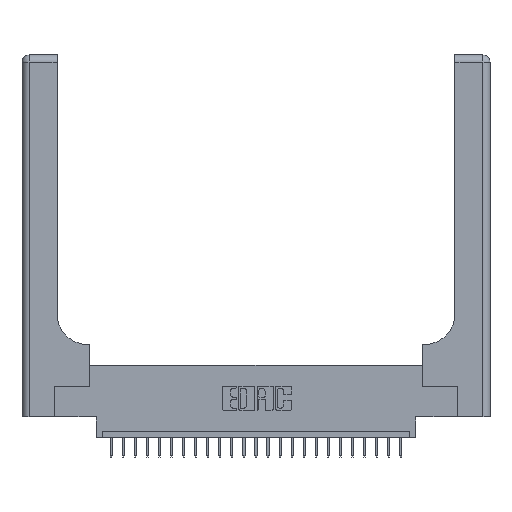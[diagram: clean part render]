
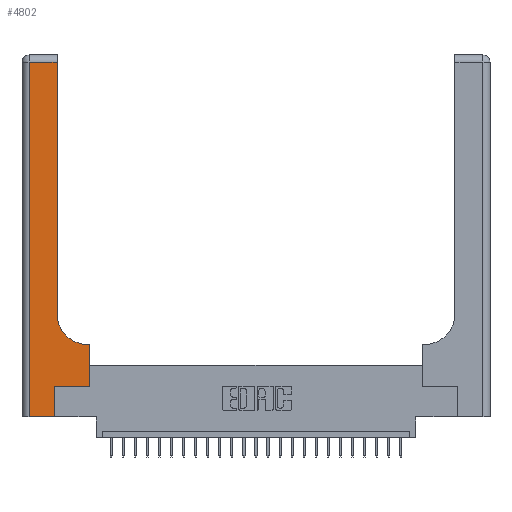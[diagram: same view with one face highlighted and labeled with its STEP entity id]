
A CAD part, top view. The second image highlights one B-rep face of the part: STEP entity #4802.
In plain terms, the highlighted planar face has unit normal (0, 0, 1).
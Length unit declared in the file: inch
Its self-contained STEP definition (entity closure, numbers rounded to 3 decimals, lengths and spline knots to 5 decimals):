
#202 = VERTEX_POINT ( 'NONE', #8876 ) ;
#686 = CARTESIAN_POINT ( 'NONE',  ( 0.06, 2.94, 0.37 ) ) ;
#2284 = DIRECTION ( 'NONE',  ( 0., 1., 0. ) ) ;
#2621 = DIRECTION ( 'NONE',  ( 0., 0., -1. ) ) ;
#2882 = PLANE ( 'NONE',  #21151 ) ;
#2911 = VERTEX_POINT ( 'NONE', #7952 ) ;
#3058 = DIRECTION ( 'NONE',  ( -1., 0., 0. ) ) ;
#3122 = ORIENTED_EDGE ( 'NONE', *, *, #18862, .T. ) ;
#3989 = VERTEX_POINT ( 'NONE', #17909 ) ;
#4230 = VERTEX_POINT ( 'NONE', #686 ) ;
#4232 = CIRCLE ( 'NONE', #15058, 0.25 ) ;
#4802 = ADVANCED_FACE ( 'NONE', ( #13613 ), #2882, .F. ) ;
#5008 = VECTOR ( 'NONE', #9974, 39.37008 ) ;
#5128 = EDGE_CURVE ( 'NONE', #3989, #202, #18696, .T. ) ;
#5741 = VERTEX_POINT ( 'NONE', #21146 ) ;
#6477 = VERTEX_POINT ( 'NONE', #24338 ) ;
#6773 = EDGE_CURVE ( 'NONE', #14384, #8627, #12584, .T. ) ;
#7535 = ORIENTED_EDGE ( 'NONE', *, *, #15723, .T. ) ;
#7834 = LINE ( 'NONE', #13498, #24083 ) ;
#7952 = CARTESIAN_POINT ( 'NONE',  ( 0.5415, 0.6, 0.37 ) ) ;
#8627 = VERTEX_POINT ( 'NONE', #24743 ) ;
#8790 = CARTESIAN_POINT ( 'NONE',  ( 0.5415, 0.85, 0.37 ) ) ;
#8876 = CARTESIAN_POINT ( 'NONE',  ( 0.5585, 0.25, 0.37 ) ) ;
#9069 = VECTOR ( 'NONE', #22063, 39.37008 ) ;
#9974 = DIRECTION ( 'NONE',  ( 0., 1., 0. ) ) ;
#10156 = VERTEX_POINT ( 'NONE', #11970 ) ;
#11117 = VECTOR ( 'NONE', #19999, 39.37008 ) ;
#11348 = VECTOR ( 'NONE', #23626, 39.37008 ) ;
#11970 = CARTESIAN_POINT ( 'NONE',  ( 0.5585, 0.6, 0.37 ) ) ;
#12013 = CARTESIAN_POINT ( 'NONE',  ( 0.06, 3., 0.37 ) ) ;
#12401 = LINE ( 'NONE', #12013, #11117 ) ;
#12412 = ORIENTED_EDGE ( 'NONE', *, *, #6773, .T. ) ;
#12584 = LINE ( 'NONE', #16720, #23110 ) ;
#13239 = CARTESIAN_POINT ( 'NONE',  ( 0., 3., 0.37 ) ) ;
#13437 = ORIENTED_EDGE ( 'NONE', *, *, #14209, .T. ) ;
#13498 = CARTESIAN_POINT ( 'NONE',  ( 0.2915, 0.6, 0.37 ) ) ;
#13613 = FACE_OUTER_BOUND ( 'NONE', #20439, .T. ) ;
#13622 = DIRECTION ( 'NONE',  ( -1., 0., 0. ) ) ;
#13705 = LINE ( 'NONE', #20097, #22325 ) ;
#14209 = EDGE_CURVE ( 'NONE', #4230, #5741, #12401, .T. ) ;
#14384 = VERTEX_POINT ( 'NONE', #24270 ) ;
#14474 = LINE ( 'NONE', #19800, #9069 ) ;
#14749 = EDGE_CURVE ( 'NONE', #6477, #3989, #19337, .T. ) ;
#14861 = ORIENTED_EDGE ( 'NONE', *, *, #26100, .T. ) ;
#14923 = LINE ( 'NONE', #21608, #23214 ) ;
#15058 = AXIS2_PLACEMENT_3D ( 'NONE', #8790, #16682, #23026 ) ;
#15723 = EDGE_CURVE ( 'NONE', #10156, #2911, #7834, .T. ) ;
#16682 = DIRECTION ( 'NONE',  ( 0., 0., -1. ) ) ;
#16720 = CARTESIAN_POINT ( 'NONE',  ( 0.2915, 3., 0.37 ) ) ;
#16881 = DIRECTION ( 'NONE',  ( -1., 0., 0. ) ) ;
#17717 = CARTESIAN_POINT ( 'NONE',  ( 0.269, 0.25, 0.37 ) ) ;
#17909 = CARTESIAN_POINT ( 'NONE',  ( 0.269, 0.25, 0.37 ) ) ;
#18056 = CARTESIAN_POINT ( 'NONE',  ( 0.269, 0., 0.37 ) ) ;
#18696 = LINE ( 'NONE', #17717, #11348 ) ;
#18862 = EDGE_CURVE ( 'NONE', #202, #10156, #14923, .T. ) ;
#19310 = ORIENTED_EDGE ( 'NONE', *, *, #24464, .T. ) ;
#19337 = LINE ( 'NONE', #18056, #5008 ) ;
#19341 = ORIENTED_EDGE ( 'NONE', *, *, #14749, .T. ) ;
#19800 = CARTESIAN_POINT ( 'NONE',  ( 0., 0., 0.37 ) ) ;
#19999 = DIRECTION ( 'NONE',  ( 0., -1., 0. ) ) ;
#20097 = CARTESIAN_POINT ( 'NONE',  ( 0., 2.94, 0.37 ) ) ;
#20268 = ORIENTED_EDGE ( 'NONE', *, *, #5128, .T. ) ;
#20439 = EDGE_LOOP ( 'NONE', ( #12412, #14861, #13437, #22741, #19341, #20268, #3122, #7535, #19310 ) ) ;
#21146 = CARTESIAN_POINT ( 'NONE',  ( 0.06, 0., 0.37 ) ) ;
#21151 = AXIS2_PLACEMENT_3D ( 'NONE', #13239, #2621, #16881 ) ;
#21608 = CARTESIAN_POINT ( 'NONE',  ( 0.5585, 0.25, 0.37 ) ) ;
#22063 = DIRECTION ( 'NONE',  ( 1., 0., 0. ) ) ;
#22325 = VECTOR ( 'NONE', #13622, 39.37008 ) ;
#22741 = ORIENTED_EDGE ( 'NONE', *, *, #23486, .T. ) ;
#23026 = DIRECTION ( 'NONE',  ( 1., 0., 0. ) ) ;
#23110 = VECTOR ( 'NONE', #2284, 39.37008 ) ;
#23214 = VECTOR ( 'NONE', #25885, 39.37008 ) ;
#23486 = EDGE_CURVE ( 'NONE', #5741, #6477, #14474, .T. ) ;
#23626 = DIRECTION ( 'NONE',  ( 1., 0., 0. ) ) ;
#24083 = VECTOR ( 'NONE', #3058, 39.37008 ) ;
#24270 = CARTESIAN_POINT ( 'NONE',  ( 0.2915, 0.85, 0.37 ) ) ;
#24338 = CARTESIAN_POINT ( 'NONE',  ( 0.269, 0., 0.37 ) ) ;
#24464 = EDGE_CURVE ( 'NONE', #2911, #14384, #4232, .T. ) ;
#24743 = CARTESIAN_POINT ( 'NONE',  ( 0.2915, 2.94, 0.37 ) ) ;
#25885 = DIRECTION ( 'NONE',  ( 0., 1., 0. ) ) ;
#26100 = EDGE_CURVE ( 'NONE', #8627, #4230, #13705, .T. ) ;
